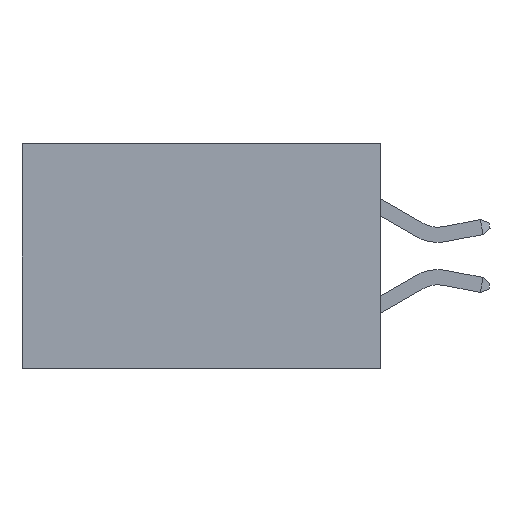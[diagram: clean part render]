
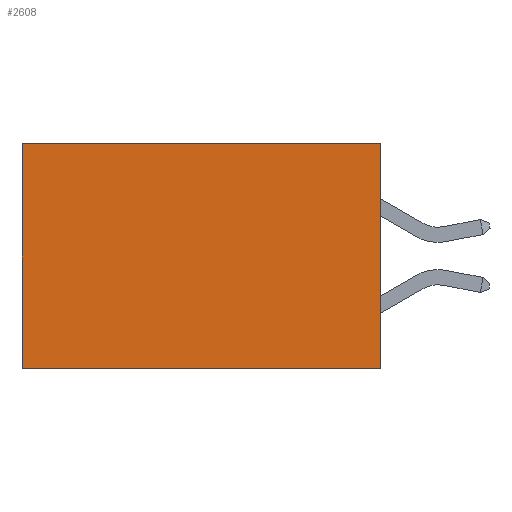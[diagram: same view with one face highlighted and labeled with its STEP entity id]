
A CAD part, left-side view. The second image highlights one B-rep face of the part: STEP entity #2608.
In plain terms, the highlighted planar face has unit normal (-1, 0, 0).
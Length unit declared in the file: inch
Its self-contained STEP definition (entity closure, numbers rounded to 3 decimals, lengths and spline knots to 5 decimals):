
#494 = EDGE_CURVE ( 'NONE', #8996, #26707, #884, .T. ) ;
#884 = LINE ( 'NONE', #20688, #27315 ) ;
#2221 = CARTESIAN_POINT ( 'NONE',  ( 0.277, 0., -0.37 ) ) ;
#2608 = ADVANCED_FACE ( 'NONE', ( #5412 ), #10625, .F. ) ;
#3525 = LINE ( 'NONE', #17510, #30686 ) ;
#4798 = ORIENTED_EDGE ( 'NONE', *, *, #494, .F. ) ;
#5412 = FACE_OUTER_BOUND ( 'NONE', #10052, .T. ) ;
#6142 = DIRECTION ( 'NONE',  ( 0., 0., -1. ) ) ;
#8996 = VERTEX_POINT ( 'NONE', #15241 ) ;
#10052 = EDGE_LOOP ( 'NONE', ( #18467, #32857, #4798, #25796 ) ) ;
#10180 = VERTEX_POINT ( 'NONE', #12153 ) ;
#10625 = PLANE ( 'NONE',  #23990 ) ;
#11412 = DIRECTION ( 'NONE',  ( 0., 1., 0. ) ) ;
#11589 = EDGE_CURVE ( 'NONE', #13049, #10180, #3525, .T. ) ;
#12153 = CARTESIAN_POINT ( 'NONE',  ( 0.277, 0.59, -0.37 ) ) ;
#12930 = CARTESIAN_POINT ( 'NONE',  ( 0.277, 0.59, 0. ) ) ;
#13049 = VERTEX_POINT ( 'NONE', #12930 ) ;
#15241 = CARTESIAN_POINT ( 'NONE',  ( 0.277, 0., 0. ) ) ;
#15699 = DIRECTION ( 'NONE',  ( 0., 0., -1. ) ) ;
#16055 = LINE ( 'NONE', #21627, #30017 ) ;
#17268 = DIRECTION ( 'NONE',  ( 1., 0., 0. ) ) ;
#17510 = CARTESIAN_POINT ( 'NONE',  ( 0.277, 0.59, -0.37 ) ) ;
#18467 = ORIENTED_EDGE ( 'NONE', *, *, #11589, .T. ) ;
#18981 = DIRECTION ( 'NONE',  ( 0., 1., 0. ) ) ;
#20688 = CARTESIAN_POINT ( 'NONE',  ( 0.277, 0., -0.37 ) ) ;
#21627 = CARTESIAN_POINT ( 'NONE',  ( 0.277, 0., -0.37 ) ) ;
#22802 = DIRECTION ( 'NONE',  ( 0., 0., -1. ) ) ;
#23990 = AXIS2_PLACEMENT_3D ( 'NONE', #33932, #17268, #15699 ) ;
#25796 = ORIENTED_EDGE ( 'NONE', *, *, #27624, .T. ) ;
#25886 = VECTOR ( 'NONE', #11412, 39.37008 ) ;
#26383 = EDGE_CURVE ( 'NONE', #26707, #10180, #16055, .T. ) ;
#26707 = VERTEX_POINT ( 'NONE', #2221 ) ;
#27054 = CARTESIAN_POINT ( 'NONE',  ( 0.277, 0., 0. ) ) ;
#27315 = VECTOR ( 'NONE', #6142, 39.37008 ) ;
#27624 = EDGE_CURVE ( 'NONE', #8996, #13049, #32806, .T. ) ;
#30017 = VECTOR ( 'NONE', #18981, 39.37008 ) ;
#30686 = VECTOR ( 'NONE', #22802, 39.37008 ) ;
#32806 = LINE ( 'NONE', #27054, #25886 ) ;
#32857 = ORIENTED_EDGE ( 'NONE', *, *, #26383, .F. ) ;
#33932 = CARTESIAN_POINT ( 'NONE',  ( 0.277, 0., -0.37 ) ) ;
